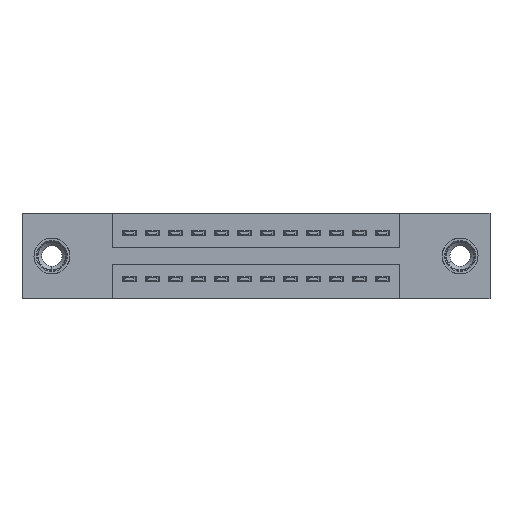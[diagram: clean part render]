
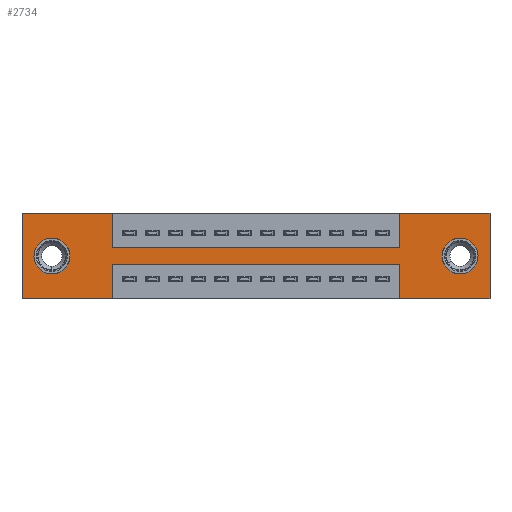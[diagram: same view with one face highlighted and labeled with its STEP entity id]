
A CAD part, front view. The second image highlights one B-rep face of the part: STEP entity #2734.
In plain terms, the highlighted planar face has unit normal (0, -1, 0).
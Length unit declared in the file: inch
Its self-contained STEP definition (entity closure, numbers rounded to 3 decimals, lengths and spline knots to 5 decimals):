
#121 = CARTESIAN_POINT ( 'NONE',  ( 0.3925, 0., -0.37 ) ) ;
#134 = VECTOR ( 'NONE', #4946, 39.37008 ) ;
#200 = ORIENTED_EDGE ( 'NONE', *, *, #12605, .F. ) ;
#480 = CARTESIAN_POINT ( 'NONE',  ( 0.3925, 0., -0.22 ) ) ;
#522 = AXIS2_PLACEMENT_3D ( 'NONE', #13637, #7926, #6950 ) ;
#792 = CARTESIAN_POINT ( 'NONE',  ( 1.905, 0., -0.263 ) ) ;
#984 = LINE ( 'NONE', #480, #10453 ) ;
#1006 = DIRECTION ( 'NONE',  ( 0., 1., 0. ) ) ;
#1058 = CARTESIAN_POINT ( 'NONE',  ( 2.035, 0., 0. ) ) ;
#1117 = VERTEX_POINT ( 'NONE', #12534 ) ;
#1200 = VERTEX_POINT ( 'NONE', #8279 ) ;
#1214 = CARTESIAN_POINT ( 'NONE',  ( 1.6425, 0., 0. ) ) ;
#1290 = VERTEX_POINT ( 'NONE', #7671 ) ;
#1312 = EDGE_CURVE ( 'NONE', #11753, #11680, #14419, .T. ) ;
#1331 = CARTESIAN_POINT ( 'NONE',  ( 1.6425, 0., -0.22 ) ) ;
#1375 = ORIENTED_EDGE ( 'NONE', *, *, #3258, .T. ) ;
#1576 = CARTESIAN_POINT ( 'NONE',  ( 1.905, 0., -0.107 ) ) ;
#1715 = CARTESIAN_POINT ( 'NONE',  ( 0.13, 0., -0.185 ) ) ;
#1840 = EDGE_CURVE ( 'NONE', #14430, #8159, #12145, .T. ) ;
#1909 = EDGE_CURVE ( 'NONE', #7518, #7353, #8148, .T. ) ;
#1941 = CARTESIAN_POINT ( 'NONE',  ( 0., 0., 0. ) ) ;
#1966 = CARTESIAN_POINT ( 'NONE',  ( 1.6425, 0., -0.37 ) ) ;
#2001 = DIRECTION ( 'NONE',  ( 1., 0., 0. ) ) ;
#2048 = AXIS2_PLACEMENT_3D ( 'NONE', #4285, #1006, #14384 ) ;
#2207 = VERTEX_POINT ( 'NONE', #121 ) ;
#2363 = DIRECTION ( 'NONE',  ( 0., -1., 0. ) ) ;
#2418 = AXIS2_PLACEMENT_3D ( 'NONE', #1715, #14093, #10622 ) ;
#2468 = VECTOR ( 'NONE', #6383, 39.37008 ) ;
#2477 = CARTESIAN_POINT ( 'NONE',  ( 0.13, 0., -0.185 ) ) ;
#2515 = ORIENTED_EDGE ( 'NONE', *, *, #4896, .F. ) ;
#2734 = ADVANCED_FACE ( 'NONE', ( #10915, #11944, #9691 ), #5542, .T. ) ;
#2767 = VERTEX_POINT ( 'NONE', #1331 ) ;
#2854 = DIRECTION ( 'NONE',  ( 0., 0., -1. ) ) ;
#3096 = VECTOR ( 'NONE', #3802, 39.37008 ) ;
#3258 = EDGE_CURVE ( 'NONE', #6332, #4105, #5954, .T. ) ;
#3353 = VECTOR ( 'NONE', #8922, 39.37008 ) ;
#3758 = VERTEX_POINT ( 'NONE', #9798 ) ;
#3802 = DIRECTION ( 'NONE',  ( 0., 0., 1. ) ) ;
#4105 = VERTEX_POINT ( 'NONE', #1576 ) ;
#4285 = CARTESIAN_POINT ( 'NONE',  ( 1.905, 0., -0.185 ) ) ;
#4314 = ORIENTED_EDGE ( 'NONE', *, *, #8535, .F. ) ;
#4584 = DIRECTION ( 'NONE',  ( 0., 0., 1. ) ) ;
#4668 = LINE ( 'NONE', #10753, #5377 ) ;
#4859 = LINE ( 'NONE', #8348, #3096 ) ;
#4896 = EDGE_CURVE ( 'NONE', #2767, #6905, #984, .T. ) ;
#4946 = DIRECTION ( 'NONE',  ( 1., 0., 0. ) ) ;
#5377 = VECTOR ( 'NONE', #10890, 39.37008 ) ;
#5422 = DIRECTION ( 'NONE',  ( 0., 0., 1. ) ) ;
#5542 = PLANE ( 'NONE',  #13136 ) ;
#5633 = AXIS2_PLACEMENT_3D ( 'NONE', #2477, #14097, #8572 ) ;
#5954 = CIRCLE ( 'NONE', #2048, 0.078 ) ;
#5956 = VECTOR ( 'NONE', #2854, 39.37008 ) ;
#6130 = ORIENTED_EDGE ( 'NONE', *, *, #1909, .F. ) ;
#6331 = ORIENTED_EDGE ( 'NONE', *, *, #13976, .F. ) ;
#6332 = VERTEX_POINT ( 'NONE', #792 ) ;
#6383 = DIRECTION ( 'NONE',  ( 0., 0., -1. ) ) ;
#6641 = ORIENTED_EDGE ( 'NONE', *, *, #11162, .F. ) ;
#6757 = CARTESIAN_POINT ( 'NONE',  ( 1.6425, 0., 0. ) ) ;
#6905 = VERTEX_POINT ( 'NONE', #10442 ) ;
#6950 = DIRECTION ( 'NONE',  ( 0., 0., -1. ) ) ;
#6981 = DIRECTION ( 'NONE',  ( 1., 0., 0. ) ) ;
#7003 = CARTESIAN_POINT ( 'NONE',  ( 0., 0., -0.37 ) ) ;
#7146 = VECTOR ( 'NONE', #6981, 39.37008 ) ;
#7353 = VERTEX_POINT ( 'NONE', #9308 ) ;
#7362 = EDGE_LOOP ( 'NONE', ( #10658, #2515, #12523, #4314, #11569, #6331, #13222, #10613, #200, #6130, #14296, #6641 ) ) ;
#7518 = VERTEX_POINT ( 'NONE', #1941 ) ;
#7671 = CARTESIAN_POINT ( 'NONE',  ( 1.6425, 0., -0.15 ) ) ;
#7873 = LINE ( 'NONE', #1966, #12401 ) ;
#7926 = DIRECTION ( 'NONE',  ( 0., 1., 0. ) ) ;
#8142 = CARTESIAN_POINT ( 'NONE',  ( 0.3925, 0., -0.15 ) ) ;
#8148 = LINE ( 'NONE', #9734, #11806 ) ;
#8159 = VERTEX_POINT ( 'NONE', #13958 ) ;
#8271 = EDGE_CURVE ( 'NONE', #1117, #7518, #4859, .T. ) ;
#8279 = CARTESIAN_POINT ( 'NONE',  ( 1.6425, 0., -0.37 ) ) ;
#8348 = CARTESIAN_POINT ( 'NONE',  ( 0., 0., 0. ) ) ;
#8409 = LINE ( 'NONE', #12555, #7146 ) ;
#8427 = ORIENTED_EDGE ( 'NONE', *, *, #11083, .T. ) ;
#8535 = EDGE_CURVE ( 'NONE', #11680, #1200, #4668, .T. ) ;
#8572 = DIRECTION ( 'NONE',  ( 0., 0., 1. ) ) ;
#8922 = DIRECTION ( 'NONE',  ( 0., 0., -1. ) ) ;
#8947 = CIRCLE ( 'NONE', #5633, 0.078 ) ;
#9100 = CARTESIAN_POINT ( 'NONE',  ( 0.13, 0., -0.263 ) ) ;
#9160 = ORIENTED_EDGE ( 'NONE', *, *, #13698, .T. ) ;
#9308 = CARTESIAN_POINT ( 'NONE',  ( 0.3925, 0., 0. ) ) ;
#9464 = EDGE_CURVE ( 'NONE', #1200, #2767, #7873, .T. ) ;
#9691 = FACE_OUTER_BOUND ( 'NONE', #7362, .T. ) ;
#9700 = EDGE_CURVE ( 'NONE', #1290, #13218, #14134, .T. ) ;
#9734 = CARTESIAN_POINT ( 'NONE',  ( 0., 0., 0. ) ) ;
#9762 = LINE ( 'NONE', #7003, #10287 ) ;
#9798 = CARTESIAN_POINT ( 'NONE',  ( 0.3925, 0., -0.15 ) ) ;
#10287 = VECTOR ( 'NONE', #13739, 39.37008 ) ;
#10365 = EDGE_CURVE ( 'NONE', #3758, #1290, #13216, .T. ) ;
#10442 = CARTESIAN_POINT ( 'NONE',  ( 0.3925, 0., -0.22 ) ) ;
#10453 = VECTOR ( 'NONE', #12720, 39.37008 ) ;
#10613 = ORIENTED_EDGE ( 'NONE', *, *, #10365, .F. ) ;
#10622 = DIRECTION ( 'NONE',  ( 0., 0., 1. ) ) ;
#10658 = ORIENTED_EDGE ( 'NONE', *, *, #11711, .F. ) ;
#10753 = CARTESIAN_POINT ( 'NONE',  ( 0., 0., -0.37 ) ) ;
#10817 = CARTESIAN_POINT ( 'NONE',  ( 0.3925, 0., -0.37 ) ) ;
#10872 = CARTESIAN_POINT ( 'NONE',  ( 0.3925, 0., 0. ) ) ;
#10890 = DIRECTION ( 'NONE',  ( -1., 0., 0. ) ) ;
#10915 = FACE_BOUND ( 'NONE', #13863, .T. ) ;
#11083 = EDGE_CURVE ( 'NONE', #4105, #6332, #13382, .T. ) ;
#11162 = EDGE_CURVE ( 'NONE', #2207, #1117, #9762, .T. ) ;
#11190 = VECTOR ( 'NONE', #4584, 39.37008 ) ;
#11394 = LINE ( 'NONE', #10872, #2468 ) ;
#11515 = CARTESIAN_POINT ( 'NONE',  ( 2.035, 0., -0.37 ) ) ;
#11569 = ORIENTED_EDGE ( 'NONE', *, *, #1312, .F. ) ;
#11680 = VERTEX_POINT ( 'NONE', #11515 ) ;
#11711 = EDGE_CURVE ( 'NONE', #6905, #2207, #12958, .T. ) ;
#11753 = VERTEX_POINT ( 'NONE', #11813 ) ;
#11806 = VECTOR ( 'NONE', #2001, 39.37008 ) ;
#11813 = CARTESIAN_POINT ( 'NONE',  ( 2.035, 0., 0. ) ) ;
#11944 = FACE_BOUND ( 'NONE', #13450, .T. ) ;
#12145 = CIRCLE ( 'NONE', #2418, 0.078 ) ;
#12401 = VECTOR ( 'NONE', #5422, 39.37008 ) ;
#12416 = DIRECTION ( 'NONE',  ( 0., 0., -1. ) ) ;
#12467 = CARTESIAN_POINT ( 'NONE',  ( 0., 0., -0.37 ) ) ;
#12523 = ORIENTED_EDGE ( 'NONE', *, *, #9464, .F. ) ;
#12534 = CARTESIAN_POINT ( 'NONE',  ( 0., 0., -0.37 ) ) ;
#12555 = CARTESIAN_POINT ( 'NONE',  ( 0., 0., 0. ) ) ;
#12605 = EDGE_CURVE ( 'NONE', #7353, #3758, #11394, .T. ) ;
#12720 = DIRECTION ( 'NONE',  ( -1., 0., 0. ) ) ;
#12846 = ORIENTED_EDGE ( 'NONE', *, *, #1840, .T. ) ;
#12958 = LINE ( 'NONE', #10817, #5956 ) ;
#13136 = AXIS2_PLACEMENT_3D ( 'NONE', #12467, #2363, #12416 ) ;
#13216 = LINE ( 'NONE', #8142, #134 ) ;
#13218 = VERTEX_POINT ( 'NONE', #1214 ) ;
#13222 = ORIENTED_EDGE ( 'NONE', *, *, #9700, .F. ) ;
#13382 = CIRCLE ( 'NONE', #522, 0.078 ) ;
#13450 = EDGE_LOOP ( 'NONE', ( #9160, #12846 ) ) ;
#13637 = CARTESIAN_POINT ( 'NONE',  ( 1.905, 0., -0.185 ) ) ;
#13698 = EDGE_CURVE ( 'NONE', #8159, #14430, #8947, .T. ) ;
#13739 = DIRECTION ( 'NONE',  ( -1., 0., 0. ) ) ;
#13863 = EDGE_LOOP ( 'NONE', ( #8427, #1375 ) ) ;
#13958 = CARTESIAN_POINT ( 'NONE',  ( 0.13, 0., -0.107 ) ) ;
#13976 = EDGE_CURVE ( 'NONE', #13218, #11753, #8409, .T. ) ;
#14093 = DIRECTION ( 'NONE',  ( 0., 1., 0. ) ) ;
#14097 = DIRECTION ( 'NONE',  ( 0., 1., 0. ) ) ;
#14134 = LINE ( 'NONE', #6757, #11190 ) ;
#14296 = ORIENTED_EDGE ( 'NONE', *, *, #8271, .F. ) ;
#14384 = DIRECTION ( 'NONE',  ( 0., 0., -1. ) ) ;
#14419 = LINE ( 'NONE', #1058, #3353 ) ;
#14430 = VERTEX_POINT ( 'NONE', #9100 ) ;
